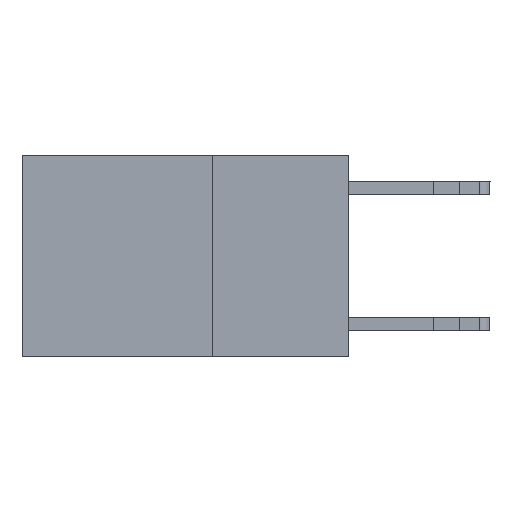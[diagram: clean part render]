
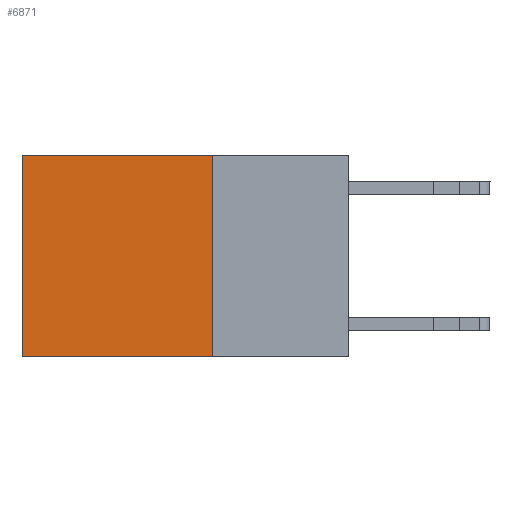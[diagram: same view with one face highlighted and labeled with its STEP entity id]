
A CAD part, left-side view. The second image highlights one B-rep face of the part: STEP entity #6871.
In plain terms, the highlighted planar face has unit normal (-1, 0, 0).
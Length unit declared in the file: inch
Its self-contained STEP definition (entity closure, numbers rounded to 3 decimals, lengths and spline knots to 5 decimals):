
#221 = VECTOR ( 'NONE', #8045, 39.37008 ) ;
#320 = CARTESIAN_POINT ( 'NONE',  ( 0.2625, 0.6, -0.37 ) ) ;
#618 = EDGE_CURVE ( 'NONE', #4293, #2445, #2494, .T. ) ;
#1106 = ORIENTED_EDGE ( 'NONE', *, *, #1208, .T. ) ;
#1208 = EDGE_CURVE ( 'NONE', #12142, #6108, #5846, .T. ) ;
#1546 = CARTESIAN_POINT ( 'NONE',  ( 0.2625, 0.6, 0. ) ) ;
#1740 = CARTESIAN_POINT ( 'NONE',  ( 0.2625, 0.25, -0.37 ) ) ;
#2445 = VERTEX_POINT ( 'NONE', #320 ) ;
#2494 = LINE ( 'NONE', #5740, #3737 ) ;
#2511 = DIRECTION ( 'NONE',  ( 0., 0., -1. ) ) ;
#2773 = DIRECTION ( 'NONE',  ( 0., 1., 0. ) ) ;
#3066 = CARTESIAN_POINT ( 'NONE',  ( 0.2625, 0.25, 0. ) ) ;
#3543 = EDGE_CURVE ( 'NONE', #6108, #2445, #11406, .T. ) ;
#3737 = VECTOR ( 'NONE', #6574, 39.37008 ) ;
#3861 = DIRECTION ( 'NONE',  ( 0., 0., -1. ) ) ;
#4293 = VERTEX_POINT ( 'NONE', #1740 ) ;
#5110 = ORIENTED_EDGE ( 'NONE', *, *, #3543, .T. ) ;
#5121 = VECTOR ( 'NONE', #2511, 39.37008 ) ;
#5424 = EDGE_CURVE ( 'NONE', #12142, #4293, #12220, .T. ) ;
#5581 = AXIS2_PLACEMENT_3D ( 'NONE', #9962, #9813, #3861 ) ;
#5740 = CARTESIAN_POINT ( 'NONE',  ( 0.2625, 0.25, -0.37 ) ) ;
#5846 = LINE ( 'NONE', #6890, #10504 ) ;
#6108 = VERTEX_POINT ( 'NONE', #1546 ) ;
#6338 = CARTESIAN_POINT ( 'NONE',  ( 0.2625, 0.6, 0. ) ) ;
#6574 = DIRECTION ( 'NONE',  ( 0., 1., 0. ) ) ;
#6871 = ADVANCED_FACE ( 'NONE', ( #7918 ), #8870, .F. ) ;
#6890 = CARTESIAN_POINT ( 'NONE',  ( 0.2625, 0.25, 0. ) ) ;
#7918 = FACE_OUTER_BOUND ( 'NONE', #11513, .T. ) ;
#8045 = DIRECTION ( 'NONE',  ( 0., 0., -1. ) ) ;
#8870 = PLANE ( 'NONE',  #5581 ) ;
#9813 = DIRECTION ( 'NONE',  ( 1., 0., 0. ) ) ;
#9962 = CARTESIAN_POINT ( 'NONE',  ( 0.2625, 0.25, 0. ) ) ;
#10504 = VECTOR ( 'NONE', #2773, 39.37008 ) ;
#11406 = LINE ( 'NONE', #6338, #5121 ) ;
#11513 = EDGE_LOOP ( 'NONE', ( #5110, #12649, #12390, #1106 ) ) ;
#12017 = CARTESIAN_POINT ( 'NONE',  ( 0.2625, 0.25, 0. ) ) ;
#12142 = VERTEX_POINT ( 'NONE', #12017 ) ;
#12220 = LINE ( 'NONE', #3066, #221 ) ;
#12390 = ORIENTED_EDGE ( 'NONE', *, *, #5424, .F. ) ;
#12649 = ORIENTED_EDGE ( 'NONE', *, *, #618, .F. ) ;
